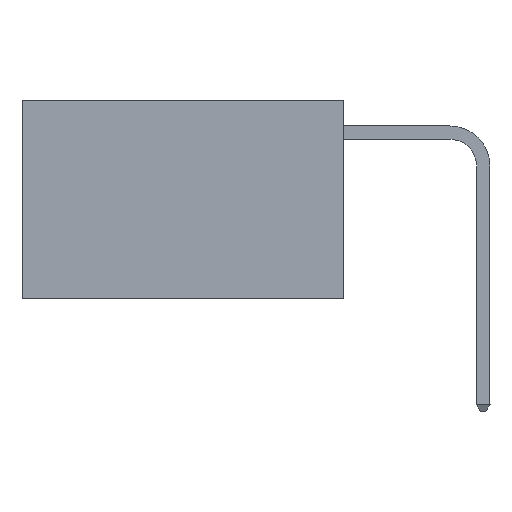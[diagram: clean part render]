
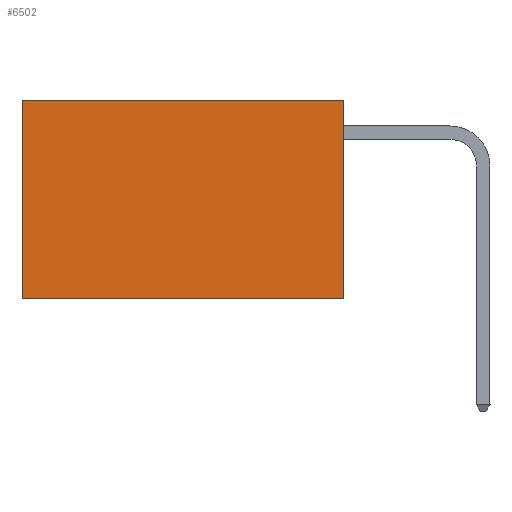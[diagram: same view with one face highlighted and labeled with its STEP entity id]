
A CAD part, left-side view. The second image highlights one B-rep face of the part: STEP entity #6502.
In plain terms, the highlighted planar face has unit normal (-1, 0, 0).
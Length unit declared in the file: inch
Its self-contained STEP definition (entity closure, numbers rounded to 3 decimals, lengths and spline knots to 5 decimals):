
#134 = ORIENTED_EDGE ( 'NONE', *, *, #20647, .F. ) ;
#641 = ORIENTED_EDGE ( 'NONE', *, *, #5218, .T. ) ;
#824 = ORIENTED_EDGE ( 'NONE', *, *, #4142, .T. ) ;
#903 = CARTESIAN_POINT ( 'NONE',  ( 0.2625, 0., 0. ) ) ;
#950 = CARTESIAN_POINT ( 'NONE',  ( 0.2625, 0., -0.37 ) ) ;
#2709 = DIRECTION ( 'NONE',  ( 1., 0., 0. ) ) ;
#3048 = LINE ( 'NONE', #11621, #11333 ) ;
#3449 = DIRECTION ( 'NONE',  ( 0., 0., -1. ) ) ;
#3982 = EDGE_CURVE ( 'NONE', #10861, #13057, #10053, .T. ) ;
#4142 = EDGE_CURVE ( 'NONE', #13436, #17566, #3048, .T. ) ;
#4750 = DIRECTION ( 'NONE',  ( 0., 0., -1. ) ) ;
#5218 = EDGE_CURVE ( 'NONE', #10861, #13436, #8199, .T. ) ;
#5551 = CARTESIAN_POINT ( 'NONE',  ( 0.2625, 0.6, 0. ) ) ;
#5576 = ORIENTED_EDGE ( 'NONE', *, *, #3982, .F. ) ;
#6165 = VECTOR ( 'NONE', #4750, 39.37008 ) ;
#6502 = ADVANCED_FACE ( 'NONE', ( #21347 ), #20901, .F. ) ;
#7968 = CARTESIAN_POINT ( 'NONE',  ( 0.2625, 0., -0.37 ) ) ;
#8199 = LINE ( 'NONE', #16025, #20407 ) ;
#10053 = LINE ( 'NONE', #13013, #6165 ) ;
#10861 = VERTEX_POINT ( 'NONE', #903 ) ;
#11333 = VECTOR ( 'NONE', #3449, 39.37008 ) ;
#11621 = CARTESIAN_POINT ( 'NONE',  ( 0.2625, 0.6, 0. ) ) ;
#12560 = DIRECTION ( 'NONE',  ( 0., 1., 0. ) ) ;
#12630 = CARTESIAN_POINT ( 'NONE',  ( 0.2625, 0., 0. ) ) ;
#13013 = CARTESIAN_POINT ( 'NONE',  ( 0.2625, 0., 0. ) ) ;
#13057 = VERTEX_POINT ( 'NONE', #7968 ) ;
#13436 = VERTEX_POINT ( 'NONE', #5551 ) ;
#13757 = EDGE_LOOP ( 'NONE', ( #824, #134, #5576, #641 ) ) ;
#13924 = AXIS2_PLACEMENT_3D ( 'NONE', #12630, #2709, #14301 ) ;
#14139 = CARTESIAN_POINT ( 'NONE',  ( 0.2625, 0.6, -0.37 ) ) ;
#14301 = DIRECTION ( 'NONE',  ( 0., 0., -1. ) ) ;
#16025 = CARTESIAN_POINT ( 'NONE',  ( 0.2625, 0., 0. ) ) ;
#16674 = VECTOR ( 'NONE', #12560, 39.37008 ) ;
#17566 = VERTEX_POINT ( 'NONE', #14139 ) ;
#17721 = DIRECTION ( 'NONE',  ( 0., 1., 0. ) ) ;
#20067 = LINE ( 'NONE', #950, #16674 ) ;
#20407 = VECTOR ( 'NONE', #17721, 39.37008 ) ;
#20647 = EDGE_CURVE ( 'NONE', #13057, #17566, #20067, .T. ) ;
#20901 = PLANE ( 'NONE',  #13924 ) ;
#21347 = FACE_OUTER_BOUND ( 'NONE', #13757, .T. ) ;
